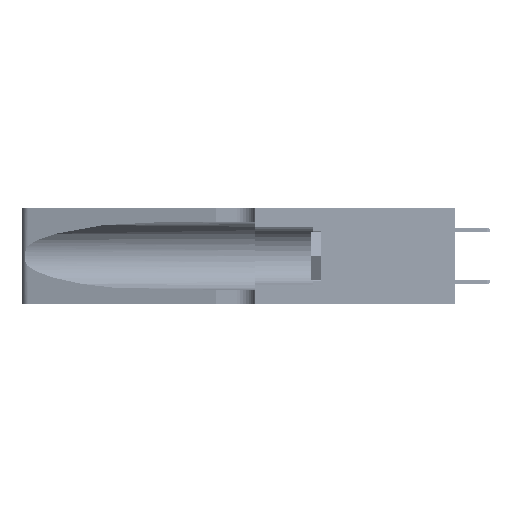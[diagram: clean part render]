
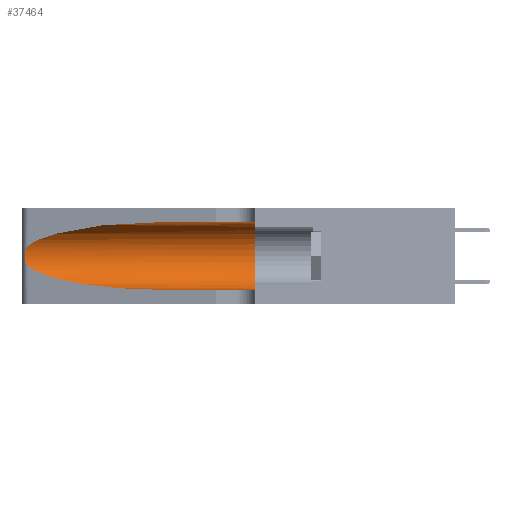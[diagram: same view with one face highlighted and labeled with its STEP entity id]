
A CAD part, left-side view. The second image highlights one B-rep face of the part: STEP entity #37464.
In plain terms, the highlighted cylindrical face has radius 3.308 mm (diameter 6.617 mm), a partial arc.
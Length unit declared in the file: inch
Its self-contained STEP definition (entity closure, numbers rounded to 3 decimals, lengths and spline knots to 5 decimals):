
#1231 = VECTOR ( 'NONE', #18674, 39.37008 ) ;
#1694 = ORIENTED_EDGE ( 'NONE', *, *, #12991, .F. ) ;
#4153 = CARTESIAN_POINT ( 'NONE',  ( 0.1305, 1.61858, 0.185 ) ) ;
#5034 = B_SPLINE_CURVE_WITH_KNOTS ( 'NONE', 3,
 ( #49650, #25945, #41527, #45116, #14742, #37465, #6610, #22390, #10163, #34134, #26466, #11177, #33643, #34384 ),
 .UNSPECIFIED., .F., .F.,
 ( 4, 2, 2, 2, 2, 2, 4 ),
 ( 0., 0.00027, 0.00053, 0.00107, 0.0016, 0.00187, 0.00214 ),
 .UNSPECIFIED. ) ;
#6330 = ORIENTED_EDGE ( 'NONE', *, *, #47289, .T. ) ;
#6610 = CARTESIAN_POINT ( 'NONE',  ( 0.26075, 1.23896, 0.19203 ) ) ;
#6613 = CARTESIAN_POINT ( 'NONE',  ( 0.25487, 1.22718, 0.14631 ) ) ;
#6727 = AXIS2_PLACEMENT_3D ( 'NONE', #13139, #9566, #25101 ) ;
#7415 = CARTESIAN_POINT ( 'NONE',  ( 0.1305, 1.61858, 0.05475 ) ) ;
#9566 = DIRECTION ( 'NONE',  ( 0., 1., 0. ) ) ;
#9746 = CARTESIAN_POINT ( 'NONE',  ( 0.1305, 1.61858, 0.31525 ) ) ;
#10097 = EDGE_LOOP ( 'NONE', ( #6330, #41879, #34965, #49391, #1694, #31797 ) ) ;
#10163 = CARTESIAN_POINT ( 'NONE',  ( 0.26017, 1.23833, 0.17102 ) ) ;
#10563 = EDGE_CURVE ( 'NONE', #36812, #14092, #25771, .T. ) ;
#11177 = CARTESIAN_POINT ( 'NONE',  ( 0.25639, 1.23186, 0.15144 ) ) ;
#11647 = CARTESIAN_POINT ( 'NONE',  ( 0.1305, 0.72297, 0.05475 ) ) ;
#12188 = DIRECTION ( 'NONE',  ( 0., 0., -1. ) ) ;
#12268 = CARTESIAN_POINT ( 'NONE',  ( 0.1305, 0.35, 0.05475 ) ) ;
#12991 = EDGE_CURVE ( 'NONE', #20923, #14092, #46611, .T. ) ;
#13139 = CARTESIAN_POINT ( 'NONE',  ( 0.1305, 0.35, 0.185 ) ) ;
#14092 = VERTEX_POINT ( 'NONE', #12268 ) ;
#14742 = CARTESIAN_POINT ( 'NONE',  ( 0.25854, 1.2359, 0.20912 ) ) ;
#16199 = VERTEX_POINT ( 'NONE', #6613 ) ;
#16230 = CARTESIAN_POINT ( 'NONE',  ( 0.18966, 0.96281, 0.31525 ) ) ;
#18674 = DIRECTION ( 'NONE',  ( 0., -1., 0. ) ) ;
#18691 = LINE ( 'NONE', #9746, #19504 ) ;
#19125 = FACE_OUTER_BOUND ( 'NONE', #10097, .T. ) ;
#19504 = VECTOR ( 'NONE', #37549, 39.37008 ) ;
#20923 = VERTEX_POINT ( 'NONE', #33444 ) ;
#22390 = CARTESIAN_POINT ( 'NONE',  ( 0.26075, 1.23896, 0.178 ) ) ;
#22833 = CARTESIAN_POINT ( 'NONE',  ( 0.2373, 1.15595, 0.08982 ) ) ;
#24128 = CARTESIAN_POINT ( 'NONE',  ( 0.1305, 0.72297, 0.31525 ) ) ;
#25101 = DIRECTION ( 'NONE',  ( 0., 0., 1. ) ) ;
#25226 = EDGE_CURVE ( 'NONE', #30245, #16199, #5034, .T. ) ;
#25771 = LINE ( 'NONE', #7415, #1231 ) ;
#25892 = CARTESIAN_POINT ( 'NONE',  ( 0.25487, 1.22718, 0.22369 ) ) ;
#25945 = CARTESIAN_POINT ( 'NONE',  ( 0.25555, 1.22994, 0.2215 ) ) ;
#26113 = AXIS2_PLACEMENT_3D ( 'NONE', #4153, #26722, #12188 ) ;
#26466 = CARTESIAN_POINT ( 'NONE',  ( 0.25789, 1.23486, 0.15765 ) ) ;
#26722 = DIRECTION ( 'NONE',  ( 0., -1., 0. ) ) ;
#27173 = VERTEX_POINT ( 'NONE', #34810 ) ;
#28200 = CARTESIAN_POINT ( 'NONE',  ( 0.2373, 1.15595, 0.28018 ) ) ;
#28686 = CARTESIAN_POINT ( 'NONE',  ( 0.25487, 1.22718, 0.22369 ) ) ;
#30245 = VERTEX_POINT ( 'NONE', #25892 ) ;
#31797 = ORIENTED_EDGE ( 'NONE', *, *, #33781, .F. ) ;
#33426 =( BOUNDED_CURVE ( )  B_SPLINE_CURVE ( 3, ( #24128, #16230, #28200, #28686 ),
 .UNSPECIFIED., .F., .T. ) 
 B_SPLINE_CURVE_WITH_KNOTS ( ( 4, 4 ),
 ( 1.5708, 2.84003 ),
 .UNSPECIFIED. ) 
 CURVE ( )  GEOMETRIC_REPRESENTATION_ITEM ( )  RATIONAL_B_SPLINE_CURVE ( ( 1., 0.87, 0.87, 1. ) ) 
 REPRESENTATION_ITEM ( '' )  );
#33444 = CARTESIAN_POINT ( 'NONE',  ( 0.1305, 0.35, 0.31525 ) ) ;
#33643 = CARTESIAN_POINT ( 'NONE',  ( 0.25555, 1.22993, 0.14849 ) ) ;
#33781 = EDGE_CURVE ( 'NONE', #27173, #20923, #18691, .T. ) ;
#34134 = CARTESIAN_POINT ( 'NONE',  ( 0.25856, 1.23593, 0.16098 ) ) ;
#34384 = CARTESIAN_POINT ( 'NONE',  ( 0.25487, 1.22718, 0.14631 ) ) ;
#34414 = CYLINDRICAL_SURFACE ( 'NONE', #26113, 0.13025 ) ;
#34810 = CARTESIAN_POINT ( 'NONE',  ( 0.1305, 0.72297, 0.31525 ) ) ;
#34965 = ORIENTED_EDGE ( 'NONE', *, *, #47140, .T. ) ;
#36812 = VERTEX_POINT ( 'NONE', #41186 ) ;
#37464 = ADVANCED_FACE ( 'NONE', ( #19125 ), #34414, .F. ) ;
#37465 = CARTESIAN_POINT ( 'NONE',  ( 0.26018, 1.23835, 0.19895 ) ) ;
#37549 = DIRECTION ( 'NONE',  ( 0., -1., 0. ) ) ;
#38171 = CARTESIAN_POINT ( 'NONE',  ( 0.25487, 1.22718, 0.14631 ) ) ;
#38421 = CARTESIAN_POINT ( 'NONE',  ( 0.18966, 0.96281, 0.05475 ) ) ;
#41186 = CARTESIAN_POINT ( 'NONE',  ( 0.1305, 0.72297, 0.05475 ) ) ;
#41527 = CARTESIAN_POINT ( 'NONE',  ( 0.25639, 1.23184, 0.21858 ) ) ;
#41879 = ORIENTED_EDGE ( 'NONE', *, *, #25226, .T. ) ;
#45116 = CARTESIAN_POINT ( 'NONE',  ( 0.25787, 1.23484, 0.2124 ) ) ;
#45404 =( BOUNDED_CURVE ( )  B_SPLINE_CURVE ( 3, ( #38171, #22833, #38421, #11647 ),
 .UNSPECIFIED., .F., .T. ) 
 B_SPLINE_CURVE_WITH_KNOTS ( ( 4, 4 ),
 ( 3.44316, 4.71239 ),
 .UNSPECIFIED. ) 
 CURVE ( )  GEOMETRIC_REPRESENTATION_ITEM ( )  RATIONAL_B_SPLINE_CURVE ( ( 1., 0.87, 0.87, 1. ) ) 
 REPRESENTATION_ITEM ( '' )  );
#46611 = CIRCLE ( 'NONE', #6727, 0.13025 ) ;
#47140 = EDGE_CURVE ( 'NONE', #16199, #36812, #45404, .T. ) ;
#47289 = EDGE_CURVE ( 'NONE', #27173, #30245, #33426, .T. ) ;
#49391 = ORIENTED_EDGE ( 'NONE', *, *, #10563, .T. ) ;
#49650 = CARTESIAN_POINT ( 'NONE',  ( 0.25487, 1.22718, 0.22369 ) ) ;
